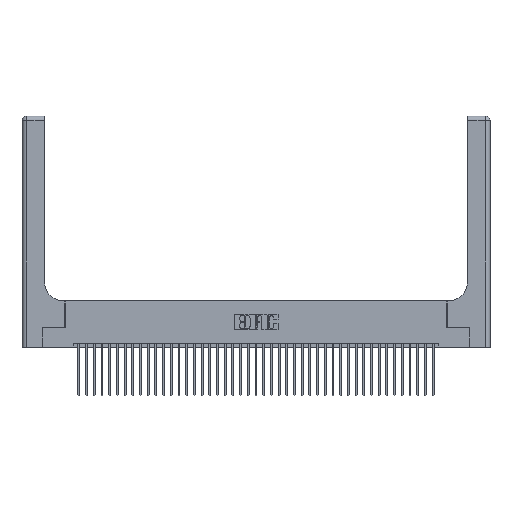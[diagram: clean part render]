
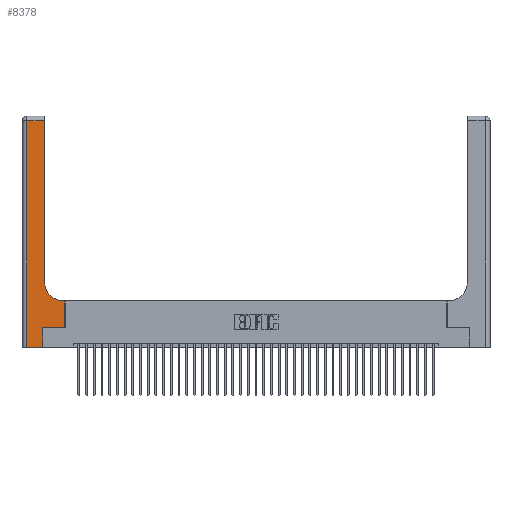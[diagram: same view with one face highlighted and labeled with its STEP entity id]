
A CAD part, top view. The second image highlights one B-rep face of the part: STEP entity #8378.
In plain terms, the highlighted planar face has unit normal (0, 0, 1).
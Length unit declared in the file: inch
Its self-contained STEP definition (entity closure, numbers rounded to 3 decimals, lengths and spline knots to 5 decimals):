
#453 = DIRECTION ( 'NONE',  ( 0., 0., -1. ) ) ;
#1525 = VECTOR ( 'NONE', #12695, 39.37008 ) ;
#1829 = CARTESIAN_POINT ( 'NONE',  ( 0.5585, 0.25, 0.37 ) ) ;
#1915 = EDGE_CURVE ( 'NONE', #18116, #34280, #27933, .T. ) ;
#1942 = CARTESIAN_POINT ( 'NONE',  ( 0., 0., 0.37 ) ) ;
#1948 = DIRECTION ( 'NONE',  ( 1., 0., 0. ) ) ;
#2310 = AXIS2_PLACEMENT_3D ( 'NONE', #40247, #21139, #1948 ) ;
#2708 = VERTEX_POINT ( 'NONE', #5954 ) ;
#4062 = ORIENTED_EDGE ( 'NONE', *, *, #19617, .T. ) ;
#4990 = ORIENTED_EDGE ( 'NONE', *, *, #37166, .T. ) ;
#5059 = DIRECTION ( 'NONE',  ( 0., 1., 0. ) ) ;
#5183 = DIRECTION ( 'NONE',  ( 1., 0., 0. ) ) ;
#5681 = ORIENTED_EDGE ( 'NONE', *, *, #18618, .T. ) ;
#5954 = CARTESIAN_POINT ( 'NONE',  ( 0.5585, 0.6, 0.37 ) ) ;
#6175 = DIRECTION ( 'NONE',  ( -1., 0., 0. ) ) ;
#6820 = VERTEX_POINT ( 'NONE', #23488 ) ;
#6946 = CARTESIAN_POINT ( 'NONE',  ( 0.269, 0.25, 0.37 ) ) ;
#7042 = VERTEX_POINT ( 'NONE', #9068 ) ;
#7800 = ORIENTED_EDGE ( 'NONE', *, *, #15246, .T. ) ;
#8378 = ADVANCED_FACE ( 'NONE', ( #15279 ), #13251, .F. ) ;
#8926 = AXIS2_PLACEMENT_3D ( 'NONE', #19663, #453, #22892 ) ;
#8943 = VERTEX_POINT ( 'NONE', #22987 ) ;
#9068 = CARTESIAN_POINT ( 'NONE',  ( 0.5585, 0.25, 0.37 ) ) ;
#9475 = CARTESIAN_POINT ( 'NONE',  ( 0.269, 0., 0.37 ) ) ;
#10118 = LINE ( 'NONE', #9475, #1525 ) ;
#10337 = LINE ( 'NONE', #15695, #18805 ) ;
#11891 = DIRECTION ( 'NONE',  ( 0., 1., 0. ) ) ;
#11902 = VECTOR ( 'NONE', #11891, 39.37008 ) ;
#12695 = DIRECTION ( 'NONE',  ( 0., 1., 0. ) ) ;
#13251 = PLANE ( 'NONE',  #8926 ) ;
#13336 = EDGE_CURVE ( 'NONE', #7042, #2708, #23511, .T. ) ;
#13495 = VECTOR ( 'NONE', #6175, 39.37008 ) ;
#13574 = EDGE_CURVE ( 'NONE', #34280, #37073, #14475, .T. ) ;
#14475 = LINE ( 'NONE', #31666, #13495 ) ;
#15027 = EDGE_CURVE ( 'NONE', #6820, #18116, #35348, .T. ) ;
#15119 = ORIENTED_EDGE ( 'NONE', *, *, #13336, .T. ) ;
#15246 = EDGE_CURVE ( 'NONE', #37739, #7042, #10337, .T. ) ;
#15279 = FACE_OUTER_BOUND ( 'NONE', #16454, .T. ) ;
#15695 = CARTESIAN_POINT ( 'NONE',  ( 0.269, 0.25, 0.37 ) ) ;
#16430 = EDGE_CURVE ( 'NONE', #19026, #37739, #10118, .T. ) ;
#16454 = EDGE_LOOP ( 'NONE', ( #34319, #34305, #4990, #4062, #18890, #7800, #15119, #5681, #20090 ) ) ;
#18116 = VERTEX_POINT ( 'NONE', #32467 ) ;
#18303 = CARTESIAN_POINT ( 'NONE',  ( 0.2915, 3., 0.37 ) ) ;
#18618 = EDGE_CURVE ( 'NONE', #2708, #6820, #36872, .T. ) ;
#18805 = VECTOR ( 'NONE', #31649, 39.37008 ) ;
#18890 = ORIENTED_EDGE ( 'NONE', *, *, #16430, .T. ) ;
#19026 = VERTEX_POINT ( 'NONE', #21609 ) ;
#19129 = LINE ( 'NONE', #35504, #35133 ) ;
#19152 = CARTESIAN_POINT ( 'NONE',  ( 0.06, 2.94, 0.37 ) ) ;
#19617 = EDGE_CURVE ( 'NONE', #8943, #19026, #25323, .T. ) ;
#19663 = CARTESIAN_POINT ( 'NONE',  ( 0., 3., 0.37 ) ) ;
#20090 = ORIENTED_EDGE ( 'NONE', *, *, #15027, .T. ) ;
#21139 = DIRECTION ( 'NONE',  ( 0., 0., -1. ) ) ;
#21609 = CARTESIAN_POINT ( 'NONE',  ( 0.269, 0., 0.37 ) ) ;
#22781 = DIRECTION ( 'NONE',  ( 0., -1., 0. ) ) ;
#22892 = DIRECTION ( 'NONE',  ( -1., 0., 0. ) ) ;
#22987 = CARTESIAN_POINT ( 'NONE',  ( 0.06, 0., 0.37 ) ) ;
#23488 = CARTESIAN_POINT ( 'NONE',  ( 0.5415, 0.6, 0.37 ) ) ;
#23511 = LINE ( 'NONE', #1829, #39477 ) ;
#25323 = LINE ( 'NONE', #1942, #41251 ) ;
#25437 = CARTESIAN_POINT ( 'NONE',  ( 0.2915, 0.6, 0.37 ) ) ;
#25582 = DIRECTION ( 'NONE',  ( -1., 0., 0. ) ) ;
#27933 = LINE ( 'NONE', #18303, #11902 ) ;
#28429 = VECTOR ( 'NONE', #25582, 39.37008 ) ;
#29591 = CARTESIAN_POINT ( 'NONE',  ( 0.2915, 2.94, 0.37 ) ) ;
#31649 = DIRECTION ( 'NONE',  ( 1., 0., 0. ) ) ;
#31666 = CARTESIAN_POINT ( 'NONE',  ( 0., 2.94, 0.37 ) ) ;
#32467 = CARTESIAN_POINT ( 'NONE',  ( 0.2915, 0.85, 0.37 ) ) ;
#34280 = VERTEX_POINT ( 'NONE', #29591 ) ;
#34305 = ORIENTED_EDGE ( 'NONE', *, *, #13574, .T. ) ;
#34319 = ORIENTED_EDGE ( 'NONE', *, *, #1915, .T. ) ;
#35133 = VECTOR ( 'NONE', #22781, 39.37008 ) ;
#35348 = CIRCLE ( 'NONE', #2310, 0.25 ) ;
#35504 = CARTESIAN_POINT ( 'NONE',  ( 0.06, 3., 0.37 ) ) ;
#36872 = LINE ( 'NONE', #25437, #28429 ) ;
#37073 = VERTEX_POINT ( 'NONE', #19152 ) ;
#37166 = EDGE_CURVE ( 'NONE', #37073, #8943, #19129, .T. ) ;
#37739 = VERTEX_POINT ( 'NONE', #6946 ) ;
#39477 = VECTOR ( 'NONE', #5059, 39.37008 ) ;
#40247 = CARTESIAN_POINT ( 'NONE',  ( 0.5415, 0.85, 0.37 ) ) ;
#41251 = VECTOR ( 'NONE', #5183, 39.37008 ) ;
